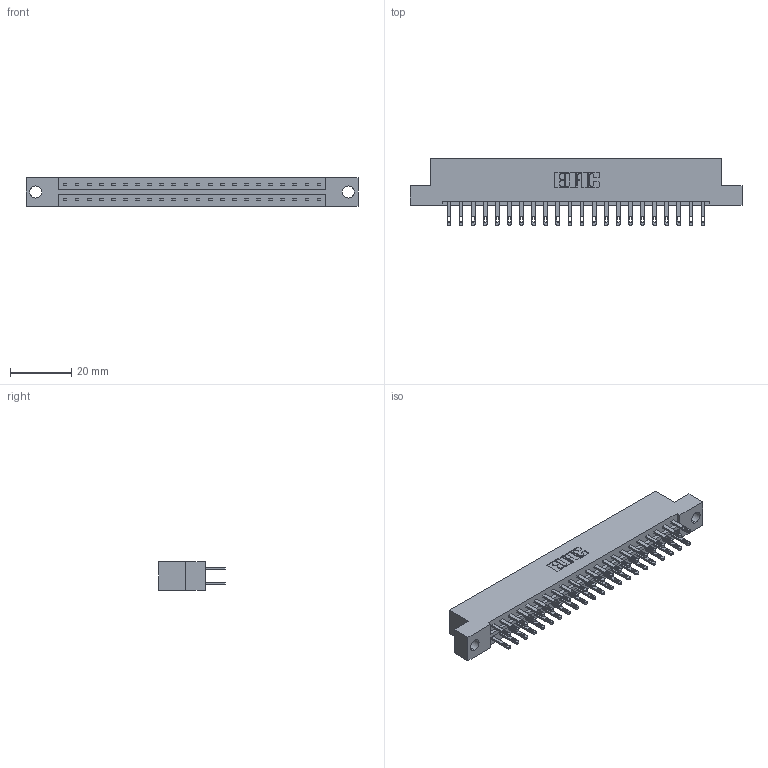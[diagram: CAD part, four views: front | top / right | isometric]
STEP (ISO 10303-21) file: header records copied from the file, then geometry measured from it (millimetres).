
FILE_DESCRIPTION (( 'STEP AP203' ), '1' );
FILE_NAME ('833-044-500-204.STEP', '2020-06-04T00:35:38', ( '' ), ( '' ), 'SwSTEP 2.0', 'SolidWorks 2020', '' );
FILE_SCHEMA (( 'CONFIG_CONTROL_DESIGN' ));
Length unit declared in the file: inch
Products named in the file (3): 833 Part_Flush - .156 Dia - TH; 345-292-001_345-293-100; 833-044-500-204
Assembly tree (45 placements, depth 2):
  833-044-500-204
    833 Part_Flush - .156 Dia - TH
    345-292-001_345-293-100  x44
Bounding box: 108.71 x 21.85 x 9.4 mm (x, y, z)
Volume: 10958.4 mm3; surface area: 13024.3 mm2
Topology: 45 solids, 45 shells, 2226 faces, 6779 edges, 4518 vertices
Faces by surface type: plane 1390, cylinder 836
Entity records: 16673 total; most frequent: CARTESIAN_POINT 2786, ORIENTED_EDGE 2722, DIRECTION 2417, EDGE_CURVE 1361, VECTOR 1229, LINE 1229, VERTEX_POINT 906, AXIS2_PLACEMENT_3D 594
